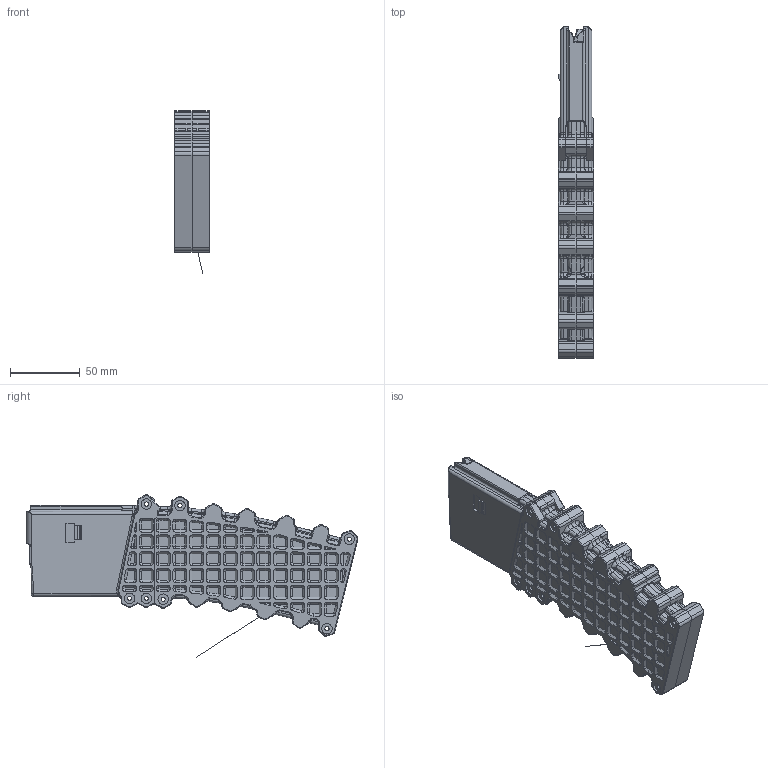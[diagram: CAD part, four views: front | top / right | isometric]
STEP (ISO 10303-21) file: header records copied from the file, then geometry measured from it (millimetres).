
FILE_DESCRIPTION (( 'STEP AP214' ), '1' );
FILE_NAME ('Extended Magazine.STEP', '2021-05-01T22:59:41', ( '' ), ( '' ), 'SwSTEP 2.0', 'SolidWorks 2020', '' );
FILE_SCHEMA (( 'AUTOMOTIVE_DESIGN' ));
Length unit declared in the file: millimetre
Products named in the file (5): Extended Magazine; Mag Body Top; Extended Mag Body Bottom Right; Extended Mag Body Bottom Left; Mag Follower
Assembly tree (4 placements, depth 2):
  Extended Magazine
    Mag Body Top
    Mag Follower
    Extended Mag Body Bottom Left
    Extended Mag Body Bottom Right
Bounding box: 25.5 x 237.2 x 116.08 mm (x, y, z)
Volume: 145076.7 mm3; surface area: 100269.1 mm2
Topology: 4 solids, 4 shells, 3879 faces, 9977 edges, 6146 vertices
Faces by surface type: plane 1281, cylinder 957, bspline 720, cone 694, torus 184, sphere 43
Entity records: 145581 total; most frequent: CARTESIAN_POINT 56475, ORIENTED_EDGE 19674, DIRECTION 17352, EDGE_CURVE 9837, AXIS2_PLACEMENT_3D 6335, VERTEX_POINT 6137, VECTOR 4682, LINE 4682
